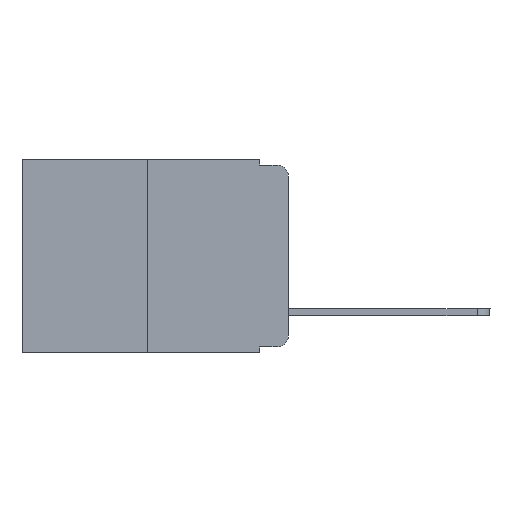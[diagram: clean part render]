
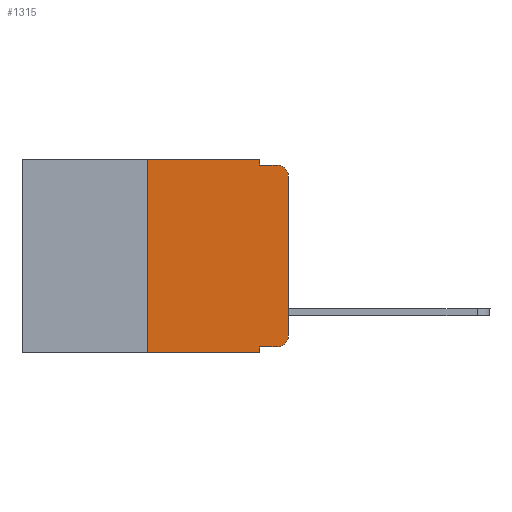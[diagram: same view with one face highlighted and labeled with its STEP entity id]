
A CAD part, left-side view. The second image highlights one B-rep face of the part: STEP entity #1315.
In plain terms, the highlighted planar face has unit normal (-1, 0, 0).
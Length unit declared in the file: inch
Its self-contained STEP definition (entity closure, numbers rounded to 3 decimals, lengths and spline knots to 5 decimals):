
#215 = VECTOR ( 'NONE', #7453, 39.37008 ) ;
#624 = VERTEX_POINT ( 'NONE', #12281 ) ;
#780 = EDGE_CURVE ( 'NONE', #624, #10813, #19881, .T. ) ;
#1065 = LINE ( 'NONE', #7420, #19230 ) ;
#1225 = DIRECTION ( 'NONE',  ( 0., 0., -1. ) ) ;
#1315 = ADVANCED_FACE ( 'NONE', ( #2799 ), #11696, .F. ) ;
#1765 = CARTESIAN_POINT ( 'NONE',  ( 0., 0.02, -0.01 ) ) ;
#1850 = AXIS2_PLACEMENT_3D ( 'NONE', #14453, #15982, #3937 ) ;
#2023 = DIRECTION ( 'NONE',  ( 0., -1., 0. ) ) ;
#2039 = VERTEX_POINT ( 'NONE', #1765 ) ;
#2063 = VERTEX_POINT ( 'NONE', #5322 ) ;
#2138 = DIRECTION ( 'NONE',  ( 0., -1., 0. ) ) ;
#2570 = ORIENTED_EDGE ( 'NONE', *, *, #4269, .F. ) ;
#2799 = FACE_OUTER_BOUND ( 'NONE', #5651, .T. ) ;
#3243 = CARTESIAN_POINT ( 'NONE',  ( 0., 0.051, 0. ) ) ;
#3471 = AXIS2_PLACEMENT_3D ( 'NONE', #13481, #15281, #1225 ) ;
#3937 = DIRECTION ( 'NONE',  ( 0., 0., -1. ) ) ;
#4265 = VERTEX_POINT ( 'NONE', #12217 ) ;
#4269 = EDGE_CURVE ( 'NONE', #2063, #15196, #1065, .T. ) ;
#4374 = EDGE_CURVE ( 'NONE', #15196, #21111, #10762, .T. ) ;
#4923 = VERTEX_POINT ( 'NONE', #21258 ) ;
#4945 = LINE ( 'NONE', #19656, #215 ) ;
#5322 = CARTESIAN_POINT ( 'NONE',  ( 0., 0.25, -0.343 ) ) ;
#5388 = EDGE_CURVE ( 'NONE', #17793, #2039, #13420, .T. ) ;
#5651 = EDGE_LOOP ( 'NONE', ( #21788, #12046, #20014, #14556, #22328, #2570, #8806, #6756, #13164, #14657 ) ) ;
#5950 = VECTOR ( 'NONE', #2138, 39.37008 ) ;
#6266 = DIRECTION ( 'NONE',  ( 0., -1., 0. ) ) ;
#6319 = EDGE_CURVE ( 'NONE', #2063, #4923, #13926, .T. ) ;
#6421 = DIRECTION ( 'NONE',  ( 0., 0., -1. ) ) ;
#6572 = CARTESIAN_POINT ( 'NONE',  ( 0., 0.051, -0.333 ) ) ;
#6756 = ORIENTED_EDGE ( 'NONE', *, *, #17116, .F. ) ;
#7420 = CARTESIAN_POINT ( 'NONE',  ( 0., 0.25, 0. ) ) ;
#7453 = DIRECTION ( 'NONE',  ( 0., 0., -1. ) ) ;
#7755 = CARTESIAN_POINT ( 'NONE',  ( 0., 0.051, -0.01 ) ) ;
#7781 = CARTESIAN_POINT ( 'NONE',  ( 0., 0.02, -0.333 ) ) ;
#8013 = CARTESIAN_POINT ( 'NONE',  ( 0., 0., -0.03 ) ) ;
#8236 = EDGE_CURVE ( 'NONE', #4265, #18967, #19325, .T. ) ;
#8806 = ORIENTED_EDGE ( 'NONE', *, *, #6319, .T. ) ;
#9166 = CARTESIAN_POINT ( 'NONE',  ( 0., 0.051, -0.01 ) ) ;
#9859 = DIRECTION ( 'NONE',  ( 1., 0., 0. ) ) ;
#10762 = LINE ( 'NONE', #12592, #15901 ) ;
#10813 = VERTEX_POINT ( 'NONE', #8013 ) ;
#11229 = DIRECTION ( 'NONE',  ( 0., -1., 0. ) ) ;
#11536 = CARTESIAN_POINT ( 'NONE',  ( 0., 0.473, 0. ) ) ;
#11696 = PLANE ( 'NONE',  #14954 ) ;
#11899 = CARTESIAN_POINT ( 'NONE',  ( 0., 0.25, 0. ) ) ;
#12046 = ORIENTED_EDGE ( 'NONE', *, *, #19339, .T. ) ;
#12217 = CARTESIAN_POINT ( 'NONE',  ( 0., 0.051, -0.333 ) ) ;
#12281 = CARTESIAN_POINT ( 'NONE',  ( 0., 0., -0.313 ) ) ;
#12592 = CARTESIAN_POINT ( 'NONE',  ( 0., 0.473, 0. ) ) ;
#12702 = CARTESIAN_POINT ( 'NONE',  ( 0., 0.473, -0.343 ) ) ;
#13164 = ORIENTED_EDGE ( 'NONE', *, *, #8236, .T. ) ;
#13420 = LINE ( 'NONE', #7755, #18372 ) ;
#13481 = CARTESIAN_POINT ( 'NONE',  ( 0., 0.02, -0.03 ) ) ;
#13926 = LINE ( 'NONE', #12702, #5950 ) ;
#14453 = CARTESIAN_POINT ( 'NONE',  ( 0., 0.02, -0.313 ) ) ;
#14556 = ORIENTED_EDGE ( 'NONE', *, *, #18268, .F. ) ;
#14657 = ORIENTED_EDGE ( 'NONE', *, *, #19620, .T. ) ;
#14954 = AXIS2_PLACEMENT_3D ( 'NONE', #11536, #9859, #6421 ) ;
#15196 = VERTEX_POINT ( 'NONE', #11899 ) ;
#15281 = DIRECTION ( 'NONE',  ( -1., 0., 0. ) ) ;
#15901 = VECTOR ( 'NONE', #2023, 39.37008 ) ;
#15982 = DIRECTION ( 'NONE',  ( -1., 0., 0. ) ) ;
#15997 = CARTESIAN_POINT ( 'NONE',  ( 0., 0.051, 0. ) ) ;
#16368 = DIRECTION ( 'NONE',  ( 0., 0., 1. ) ) ;
#16639 = CIRCLE ( 'NONE', #3471, 0.02 ) ;
#17116 = EDGE_CURVE ( 'NONE', #4265, #4923, #4945, .T. ) ;
#17135 = VECTOR ( 'NONE', #6266, 39.37008 ) ;
#17465 = DIRECTION ( 'NONE',  ( 0., 0., -1. ) ) ;
#17793 = VERTEX_POINT ( 'NONE', #9166 ) ;
#18060 = CARTESIAN_POINT ( 'NONE',  ( 0., 0., 0. ) ) ;
#18268 = EDGE_CURVE ( 'NONE', #21111, #17793, #19736, .T. ) ;
#18372 = VECTOR ( 'NONE', #11229, 39.37008 ) ;
#18756 = VECTOR ( 'NONE', #16368, 39.37008 ) ;
#18967 = VERTEX_POINT ( 'NONE', #7781 ) ;
#19230 = VECTOR ( 'NONE', #19624, 39.37008 ) ;
#19325 = LINE ( 'NONE', #6572, #17135 ) ;
#19339 = EDGE_CURVE ( 'NONE', #10813, #2039, #16639, .T. ) ;
#19620 = EDGE_CURVE ( 'NONE', #18967, #624, #20501, .T. ) ;
#19624 = DIRECTION ( 'NONE',  ( 0., 0., 1. ) ) ;
#19656 = CARTESIAN_POINT ( 'NONE',  ( 0., 0.051, 0. ) ) ;
#19736 = LINE ( 'NONE', #15997, #21116 ) ;
#19881 = LINE ( 'NONE', #18060, #18756 ) ;
#20014 = ORIENTED_EDGE ( 'NONE', *, *, #5388, .F. ) ;
#20501 = CIRCLE ( 'NONE', #1850, 0.02 ) ;
#21111 = VERTEX_POINT ( 'NONE', #3243 ) ;
#21116 = VECTOR ( 'NONE', #17465, 39.37008 ) ;
#21258 = CARTESIAN_POINT ( 'NONE',  ( 0., 0.051, -0.343 ) ) ;
#21788 = ORIENTED_EDGE ( 'NONE', *, *, #780, .T. ) ;
#22328 = ORIENTED_EDGE ( 'NONE', *, *, #4374, .F. ) ;
